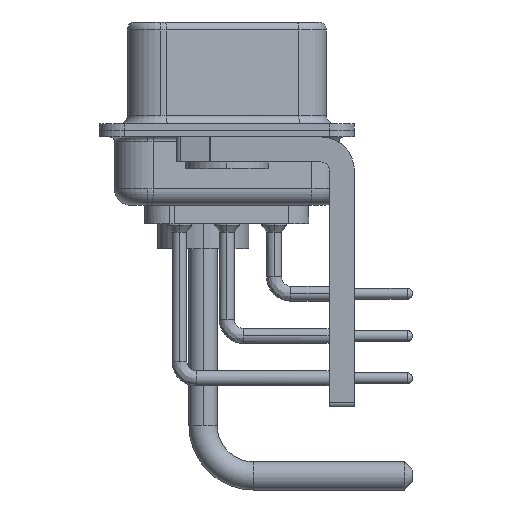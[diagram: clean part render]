
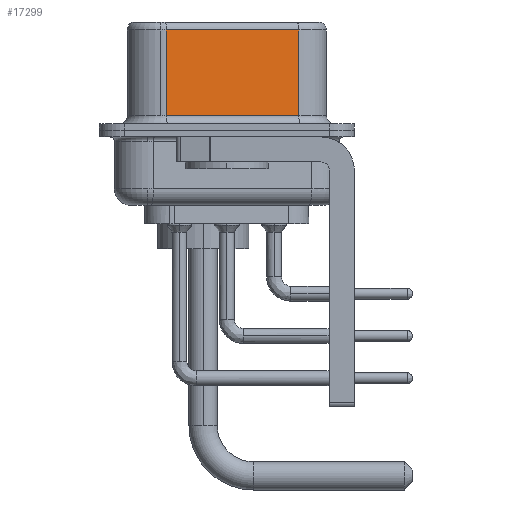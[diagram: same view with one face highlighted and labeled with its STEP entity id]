
A CAD part, left-side view. The second image highlights one B-rep face of the part: STEP entity #17299.
In plain terms, the highlighted planar face has unit normal (-0.985, -0.174, 0).
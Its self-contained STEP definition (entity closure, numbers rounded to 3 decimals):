
#1486 = VERTEX_POINT ( 'NONE', #32992 ) ;
#1831 = DIRECTION ( 'NONE',  ( 0., 0., -1. ) ) ;
#1890 = VECTOR ( 'NONE', #9511, 1000. ) ;
#2149 = DIRECTION ( 'NONE',  ( 0.174, -0.985, 0. ) ) ;
#2951 = FACE_OUTER_BOUND ( 'NONE', #11227, .T. ) ;
#4888 = VERTEX_POINT ( 'NONE', #6128 ) ;
#6128 = CARTESIAN_POINT ( 'NONE',  ( 5.132, -4.322, 6.02 ) ) ;
#6909 = CARTESIAN_POINT ( 'NONE',  ( 5.132, -4.322, 6.52 ) ) ;
#8103 = EDGE_CURVE ( 'NONE', #22072, #35665, #15501, .T. ) ;
#9511 = DIRECTION ( 'NONE',  ( -0.174, 0.985, 0. ) ) ;
#9715 = LINE ( 'NONE', #6909, #10549 ) ;
#10444 = CARTESIAN_POINT ( 'NONE',  ( 3.73, 3.628, 6.52 ) ) ;
#10549 = VECTOR ( 'NONE', #30487, 1000. ) ;
#11227 = EDGE_LOOP ( 'NONE', ( #24443, #13824, #16041, #20496 ) ) ;
#11935 = PLANE ( 'NONE',  #36543 ) ;
#12323 = CARTESIAN_POINT ( 'NONE',  ( 5.132, -4.322, 6.02 ) ) ;
#13824 = ORIENTED_EDGE ( 'NONE', *, *, #28107, .T. ) ;
#14385 = DIRECTION ( 'NONE',  ( 0.985, 0.174, 0. ) ) ;
#15129 = LINE ( 'NONE', #12323, #1890 ) ;
#15501 = LINE ( 'NONE', #10444, #36006 ) ;
#16041 = ORIENTED_EDGE ( 'NONE', *, *, #8103, .T. ) ;
#16392 = LINE ( 'NONE', #27783, #24976 ) ;
#17299 = ADVANCED_FACE ( 'NONE', ( #2951 ), #11935, .F. ) ;
#20496 = ORIENTED_EDGE ( 'NONE', *, *, #36695, .T. ) ;
#20518 = CARTESIAN_POINT ( 'NONE',  ( 5.132, -4.322, 6.52 ) ) ;
#21909 = EDGE_CURVE ( 'NONE', #4888, #1486, #9715, .T. ) ;
#22072 = VERTEX_POINT ( 'NONE', #36840 ) ;
#24443 = ORIENTED_EDGE ( 'NONE', *, *, #21909, .F. ) ;
#24976 = VECTOR ( 'NONE', #2149, 1000. ) ;
#27783 = CARTESIAN_POINT ( 'NONE',  ( 5.132, -4.322, 0.9 ) ) ;
#28107 = EDGE_CURVE ( 'NONE', #4888, #22072, #15129, .T. ) ;
#30487 = DIRECTION ( 'NONE',  ( 0., 0., -1. ) ) ;
#32992 = CARTESIAN_POINT ( 'NONE',  ( 5.132, -4.322, 0.9 ) ) ;
#34947 = DIRECTION ( 'NONE',  ( -0.174, 0.985, 0. ) ) ;
#35610 = CARTESIAN_POINT ( 'NONE',  ( 3.73, 3.628, 0.9 ) ) ;
#35665 = VERTEX_POINT ( 'NONE', #35610 ) ;
#36006 = VECTOR ( 'NONE', #1831, 1000. ) ;
#36543 = AXIS2_PLACEMENT_3D ( 'NONE', #20518, #14385, #34947 ) ;
#36695 = EDGE_CURVE ( 'NONE', #35665, #1486, #16392, .T. ) ;
#36840 = CARTESIAN_POINT ( 'NONE',  ( 3.73, 3.628, 6.02 ) ) ;
